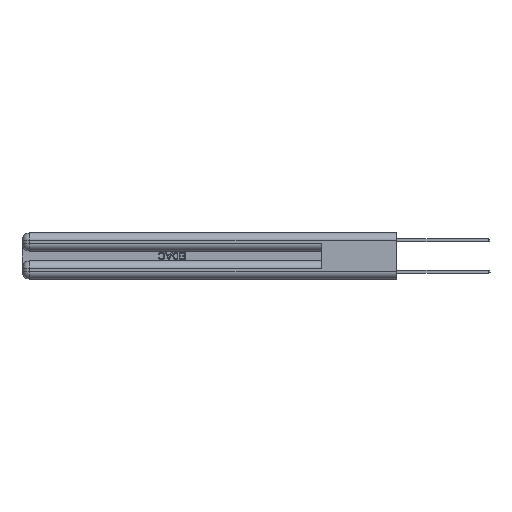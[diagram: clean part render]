
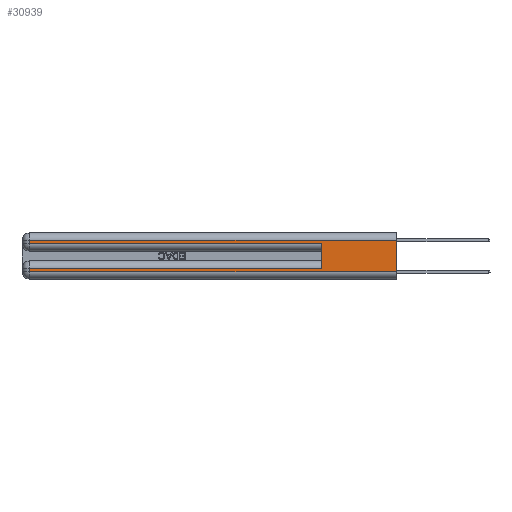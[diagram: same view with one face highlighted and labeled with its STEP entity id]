
A CAD part, left-side view. The second image highlights one B-rep face of the part: STEP entity #30939.
In plain terms, the highlighted planar face has unit normal (-1, 0, 0).
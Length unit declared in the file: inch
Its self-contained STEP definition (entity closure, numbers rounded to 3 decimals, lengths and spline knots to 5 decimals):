
#60 = ORIENTED_EDGE ( 'NONE', *, *, #3513, .T. ) ;
#340 = VERTEX_POINT ( 'NONE', #31643 ) ;
#1521 = ORIENTED_EDGE ( 'NONE', *, *, #24250, .T. ) ;
#2206 = VECTOR ( 'NONE', #29383, 39.37008 ) ;
#2746 = ORIENTED_EDGE ( 'NONE', *, *, #32348, .F. ) ;
#3275 = CARTESIAN_POINT ( 'NONE',  ( 0., 2.94, 0.085 ) ) ;
#3312 = CARTESIAN_POINT ( 'NONE',  ( 0., 2.94, 0.37 ) ) ;
#3513 = EDGE_CURVE ( 'NONE', #29926, #18772, #32575, .T. ) ;
#3556 = VERTEX_POINT ( 'NONE', #8387 ) ;
#3573 = CARTESIAN_POINT ( 'NONE',  ( 0., 0.6, 0.145 ) ) ;
#3769 = DIRECTION ( 'NONE',  ( 1., 0., 0. ) ) ;
#3975 = LINE ( 'NONE', #3312, #33657 ) ;
#4948 = VECTOR ( 'NONE', #14369, 39.37008 ) ;
#5428 = EDGE_CURVE ( 'NONE', #10917, #13246, #22917, .T. ) ;
#7886 = EDGE_CURVE ( 'NONE', #29926, #3556, #23593, .T. ) ;
#8387 = CARTESIAN_POINT ( 'NONE',  ( 0., 0.6, 0.285 ) ) ;
#10533 = LINE ( 'NONE', #11679, #16998 ) ;
#10917 = VERTEX_POINT ( 'NONE', #11847 ) ;
#11257 = CARTESIAN_POINT ( 'NONE',  ( 0., 2.94, 0.285 ) ) ;
#11320 = LINE ( 'NONE', #19138, #28378 ) ;
#11395 = ORIENTED_EDGE ( 'NONE', *, *, #24068, .T. ) ;
#11540 = DIRECTION ( 'NONE',  ( 0., 0., 1. ) ) ;
#11679 = CARTESIAN_POINT ( 'NONE',  ( 0., 0., 0.31 ) ) ;
#11737 = DIRECTION ( 'NONE',  ( 0., 0., -1. ) ) ;
#11847 = CARTESIAN_POINT ( 'NONE',  ( 0., 2.94, 0.06 ) ) ;
#11854 = PLANE ( 'NONE',  #22007 ) ;
#12258 = CARTESIAN_POINT ( 'NONE',  ( 0., 0., 0.06 ) ) ;
#13246 = VERTEX_POINT ( 'NONE', #12258 ) ;
#13502 = DIRECTION ( 'NONE',  ( 0., 1., 0. ) ) ;
#14369 = DIRECTION ( 'NONE',  ( 0., 0., -1. ) ) ;
#15017 = VECTOR ( 'NONE', #11540, 39.37008 ) ;
#16998 = VECTOR ( 'NONE', #24753, 39.37008 ) ;
#17126 = LINE ( 'NONE', #22554, #4948 ) ;
#17521 = DIRECTION ( 'NONE',  ( 0., 0., -1. ) ) ;
#18772 = VERTEX_POINT ( 'NONE', #3275 ) ;
#19138 = CARTESIAN_POINT ( 'NONE',  ( 0., 2.94, 0.37 ) ) ;
#19374 = CARTESIAN_POINT ( 'NONE',  ( 0., 0., 0.06 ) ) ;
#19552 = ORIENTED_EDGE ( 'NONE', *, *, #22762, .T. ) ;
#21039 = VECTOR ( 'NONE', #22525, 39.37008 ) ;
#21366 = ORIENTED_EDGE ( 'NONE', *, *, #7886, .F. ) ;
#21590 = DIRECTION ( 'NONE',  ( 0., 0., -1. ) ) ;
#22007 = AXIS2_PLACEMENT_3D ( 'NONE', #32738, #3769, #11737 ) ;
#22525 = DIRECTION ( 'NONE',  ( 0., -1., 0. ) ) ;
#22554 = CARTESIAN_POINT ( 'NONE',  ( 0., 0., 0.37 ) ) ;
#22666 = VERTEX_POINT ( 'NONE', #30072 ) ;
#22762 = EDGE_CURVE ( 'NONE', #22666, #340, #10533, .T. ) ;
#22917 = LINE ( 'NONE', #19374, #2206 ) ;
#23096 = VERTEX_POINT ( 'NONE', #11257 ) ;
#23593 = LINE ( 'NONE', #3573, #15017 ) ;
#24068 = EDGE_CURVE ( 'NONE', #340, #23096, #11320, .T. ) ;
#24212 = ORIENTED_EDGE ( 'NONE', *, *, #28122, .T. ) ;
#24250 = EDGE_CURVE ( 'NONE', #18772, #10917, #3975, .T. ) ;
#24753 = DIRECTION ( 'NONE',  ( 0., 1., 0. ) ) ;
#25056 = CARTESIAN_POINT ( 'NONE',  ( 0., 0., 0.285 ) ) ;
#25683 = VECTOR ( 'NONE', #13502, 39.37008 ) ;
#26617 = ORIENTED_EDGE ( 'NONE', *, *, #5428, .T. ) ;
#28122 = EDGE_CURVE ( 'NONE', #23096, #3556, #29581, .T. ) ;
#28378 = VECTOR ( 'NONE', #17521, 39.37008 ) ;
#29144 = EDGE_LOOP ( 'NONE', ( #2746, #19552, #11395, #24212, #21366, #60, #1521, #26617 ) ) ;
#29383 = DIRECTION ( 'NONE',  ( 0., -1., 0. ) ) ;
#29581 = LINE ( 'NONE', #25056, #21039 ) ;
#29926 = VERTEX_POINT ( 'NONE', #32840 ) ;
#30072 = CARTESIAN_POINT ( 'NONE',  ( 0., 0., 0.31 ) ) ;
#30625 = FACE_OUTER_BOUND ( 'NONE', #29144, .T. ) ;
#30927 = CARTESIAN_POINT ( 'NONE',  ( 0., 0., 0.085 ) ) ;
#30939 = ADVANCED_FACE ( 'NONE', ( #30625 ), #11854, .F. ) ;
#31643 = CARTESIAN_POINT ( 'NONE',  ( 0., 2.94, 0.31 ) ) ;
#32348 = EDGE_CURVE ( 'NONE', #22666, #13246, #17126, .T. ) ;
#32575 = LINE ( 'NONE', #30927, #25683 ) ;
#32738 = CARTESIAN_POINT ( 'NONE',  ( 0., 0., 0.37 ) ) ;
#32840 = CARTESIAN_POINT ( 'NONE',  ( 0., 0.6, 0.085 ) ) ;
#33657 = VECTOR ( 'NONE', #21590, 39.37008 ) ;
